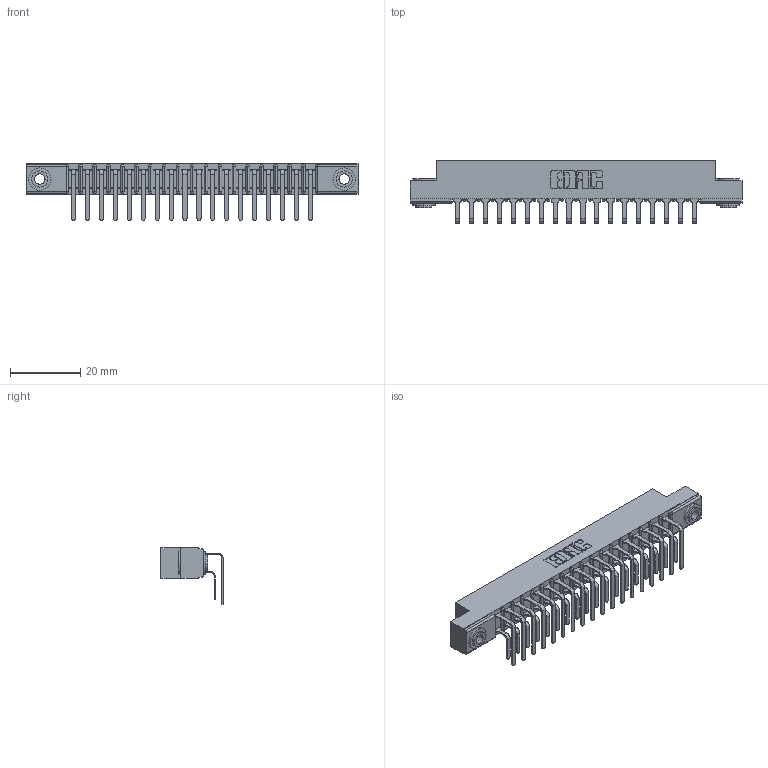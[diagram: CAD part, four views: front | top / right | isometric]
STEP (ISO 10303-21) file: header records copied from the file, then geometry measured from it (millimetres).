
FILE_DESCRIPTION (( 'STEP AP203' ), '1' );
FILE_NAME ('357-036-459-203.STEP', '2020-10-03T18:18:18', ( '' ), ( '' ), 'SwSTEP 2.0', 'SolidWorks 2020', '' );
FILE_SCHEMA (( 'CONFIG_CONTROL_DESIGN' ));
Length unit declared in the file: inch
Products named in the file (5): 357-036-459-203; 345-250-002_345-250-002-102; 307-290-001_558 559 - 1 (Single); 307 Part_.156 Dia Mounting Holes; 307-290-001_559 - 2 (Single)
Assembly tree (39 placements, depth 2):
  357-036-459-203
    307 Part_.156 Dia Mounting Holes
    307-290-001_558 559 - 1 (Single)  x18
    307-290-001_559 - 2 (Single)  x18
    345-250-002_345-250-002-102  x2
Bounding box: 94.34 x 17.69 x 16.08 mm (x, y, z)
Volume: 6331.9 mm3; surface area: 12120.8 mm2
Topology: 39 solids, 39 shells, 1989 faces, 5547 edges, 3594 vertices
Faces by surface type: plane 1282, cylinder 661, sphere 38, cone 8
Entity records: 21478 total; most frequent: CARTESIAN_POINT 3505, ORIENTED_EDGE 3462, DIRECTION 3457, EDGE_CURVE 1731, LINE 1309, VECTOR 1309, VERTEX_POINT 1122, AXIS2_PLACEMENT_3D 1074
